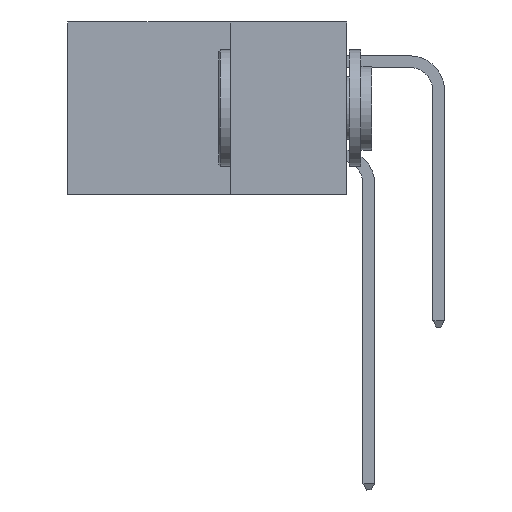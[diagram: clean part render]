
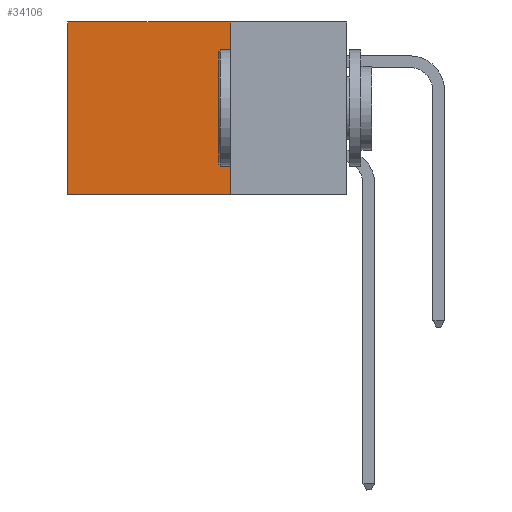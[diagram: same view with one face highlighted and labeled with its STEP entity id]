
A CAD part, left-side view. The second image highlights one B-rep face of the part: STEP entity #34106.
In plain terms, the highlighted planar face has unit normal (-1, 0, 0).
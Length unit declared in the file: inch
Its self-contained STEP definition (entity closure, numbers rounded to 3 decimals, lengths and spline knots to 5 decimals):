
#431 = DIRECTION ( 'NONE',  ( 0., 0., -1. ) ) ;
#1414 = LINE ( 'NONE', #27891, #10462 ) ;
#3079 = LINE ( 'NONE', #27332, #31389 ) ;
#3096 = VECTOR ( 'NONE', #18731, 39.37008 ) ;
#4422 = VERTEX_POINT ( 'NONE', #34563 ) ;
#4452 = LINE ( 'NONE', #7172, #3096 ) ;
#5135 = EDGE_LOOP ( 'NONE', ( #31664, #28759, #16118, #32272 ) ) ;
#5999 = CARTESIAN_POINT ( 'NONE',  ( 0.2875, 0.6, 0. ) ) ;
#6791 = EDGE_CURVE ( 'NONE', #30189, #8036, #3079, .T. ) ;
#7172 = CARTESIAN_POINT ( 'NONE',  ( 0.2875, 0.25, 0. ) ) ;
#7416 = FACE_OUTER_BOUND ( 'NONE', #5135, .T. ) ;
#8036 = VERTEX_POINT ( 'NONE', #13575 ) ;
#9242 = PLANE ( 'NONE',  #33785 ) ;
#9356 = VERTEX_POINT ( 'NONE', #33327 ) ;
#10462 = VECTOR ( 'NONE', #34159, 39.37008 ) ;
#10843 = EDGE_CURVE ( 'NONE', #9356, #8036, #20402, .T. ) ;
#11773 = DIRECTION ( 'NONE',  ( 0., 0., -1. ) ) ;
#13575 = CARTESIAN_POINT ( 'NONE',  ( 0.2875, 0.6, -0.37 ) ) ;
#14896 = DIRECTION ( 'NONE',  ( 1., 0., 0. ) ) ;
#16118 = ORIENTED_EDGE ( 'NONE', *, *, #35760, .F. ) ;
#18430 = DIRECTION ( 'NONE',  ( 0., 1., 0. ) ) ;
#18731 = DIRECTION ( 'NONE',  ( 0., 1., 0. ) ) ;
#20265 = CARTESIAN_POINT ( 'NONE',  ( 0.2875, 0.25, 0. ) ) ;
#20402 = LINE ( 'NONE', #5999, #28452 ) ;
#24280 = CARTESIAN_POINT ( 'NONE',  ( 0.2875, 0.25, -0.37 ) ) ;
#27332 = CARTESIAN_POINT ( 'NONE',  ( 0.2875, 0.25, -0.37 ) ) ;
#27382 = EDGE_CURVE ( 'NONE', #4422, #9356, #4452, .T. ) ;
#27891 = CARTESIAN_POINT ( 'NONE',  ( 0.2875, 0.25, 0. ) ) ;
#28452 = VECTOR ( 'NONE', #431, 39.37008 ) ;
#28759 = ORIENTED_EDGE ( 'NONE', *, *, #6791, .F. ) ;
#30189 = VERTEX_POINT ( 'NONE', #24280 ) ;
#31389 = VECTOR ( 'NONE', #18430, 39.37008 ) ;
#31664 = ORIENTED_EDGE ( 'NONE', *, *, #10843, .T. ) ;
#32272 = ORIENTED_EDGE ( 'NONE', *, *, #27382, .T. ) ;
#33327 = CARTESIAN_POINT ( 'NONE',  ( 0.2875, 0.6, 0. ) ) ;
#33785 = AXIS2_PLACEMENT_3D ( 'NONE', #20265, #14896, #11773 ) ;
#34106 = ADVANCED_FACE ( 'NONE', ( #7416 ), #9242, .F. ) ;
#34159 = DIRECTION ( 'NONE',  ( 0., 0., -1. ) ) ;
#34563 = CARTESIAN_POINT ( 'NONE',  ( 0.2875, 0.25, 0. ) ) ;
#35760 = EDGE_CURVE ( 'NONE', #4422, #30189, #1414, .T. ) ;
